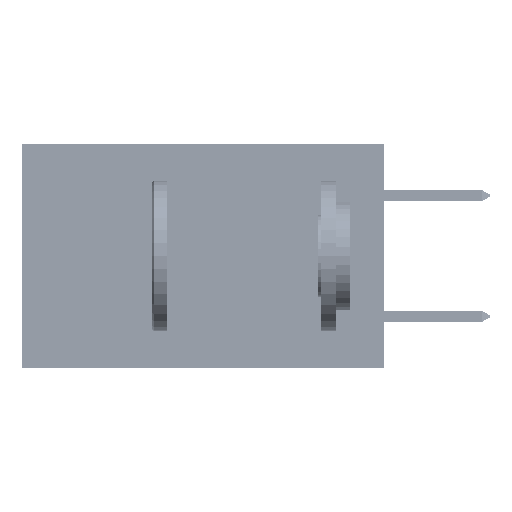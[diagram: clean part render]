
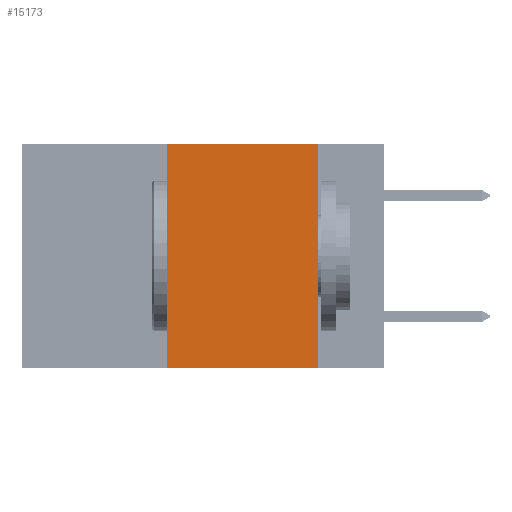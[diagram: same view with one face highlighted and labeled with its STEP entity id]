
A CAD part, left-side view. The second image highlights one B-rep face of the part: STEP entity #15173.
In plain terms, the highlighted planar face has unit normal (-1, 0, 0).
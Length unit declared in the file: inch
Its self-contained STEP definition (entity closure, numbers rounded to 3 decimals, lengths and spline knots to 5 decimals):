
#356 = DIRECTION ( 'NONE',  ( 0., -1., 0. ) ) ;
#526 = VERTEX_POINT ( 'NONE', #47827 ) ;
#812 = LINE ( 'NONE', #11266, #9826 ) ;
#2956 = DIRECTION ( 'NONE',  ( 1., 0., 0. ) ) ;
#6276 = CARTESIAN_POINT ( 'NONE',  ( 0., 0.11, 0. ) ) ;
#6877 = CARTESIAN_POINT ( 'NONE',  ( 0., 0.36, -0.37 ) ) ;
#7892 = CARTESIAN_POINT ( 'NONE',  ( 0., 0.36, 0. ) ) ;
#9153 = EDGE_LOOP ( 'NONE', ( #14280, #36942, #21425, #44081 ) ) ;
#9826 = VECTOR ( 'NONE', #30258, 39.37008 ) ;
#11266 = CARTESIAN_POINT ( 'NONE',  ( 0., 0.36, 0. ) ) ;
#11793 = CARTESIAN_POINT ( 'NONE',  ( 0., 0.6, 0. ) ) ;
#12026 = VERTEX_POINT ( 'NONE', #7892 ) ;
#14280 = ORIENTED_EDGE ( 'NONE', *, *, #24437, .F. ) ;
#14413 = PLANE ( 'NONE',  #49445 ) ;
#14960 = VERTEX_POINT ( 'NONE', #23851 ) ;
#15173 = ADVANCED_FACE ( 'NONE', ( #32003 ), #14413, .F. ) ;
#21425 = ORIENTED_EDGE ( 'NONE', *, *, #42659, .F. ) ;
#21895 = DIRECTION ( 'NONE',  ( 0., -1., 0. ) ) ;
#22363 = VECTOR ( 'NONE', #356, 39.37008 ) ;
#23851 = CARTESIAN_POINT ( 'NONE',  ( 0., 0.11, -0.37 ) ) ;
#24437 = EDGE_CURVE ( 'NONE', #526, #14960, #43521, .T. ) ;
#25857 = CARTESIAN_POINT ( 'NONE',  ( 0., 0.6, 0. ) ) ;
#27288 = EDGE_CURVE ( 'NONE', #46510, #14960, #40066, .T. ) ;
#29188 = DIRECTION ( 'NONE',  ( 0., 0., -1. ) ) ;
#29715 = DIRECTION ( 'NONE',  ( 0., 0., -1. ) ) ;
#29899 = VECTOR ( 'NONE', #21895, 39.37008 ) ;
#30258 = DIRECTION ( 'NONE',  ( 0., 0., 1. ) ) ;
#31009 = EDGE_CURVE ( 'NONE', #12026, #526, #33722, .T. ) ;
#32003 = FACE_OUTER_BOUND ( 'NONE', #9153, .T. ) ;
#33576 = CARTESIAN_POINT ( 'NONE',  ( 0., 0.6, -0.37 ) ) ;
#33722 = LINE ( 'NONE', #11793, #22363 ) ;
#34615 = VECTOR ( 'NONE', #29188, 39.37008 ) ;
#36942 = ORIENTED_EDGE ( 'NONE', *, *, #31009, .F. ) ;
#40066 = LINE ( 'NONE', #33576, #29899 ) ;
#42659 = EDGE_CURVE ( 'NONE', #46510, #12026, #812, .T. ) ;
#43521 = LINE ( 'NONE', #6276, #34615 ) ;
#44081 = ORIENTED_EDGE ( 'NONE', *, *, #27288, .T. ) ;
#46510 = VERTEX_POINT ( 'NONE', #6877 ) ;
#47827 = CARTESIAN_POINT ( 'NONE',  ( 0., 0.11, 0. ) ) ;
#49445 = AXIS2_PLACEMENT_3D ( 'NONE', #25857, #2956, #29715 ) ;
